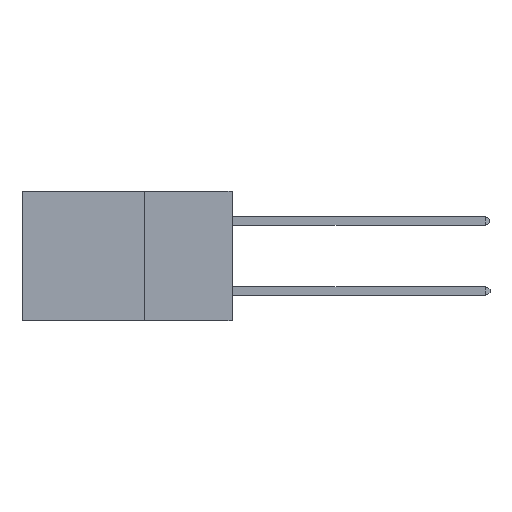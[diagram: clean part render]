
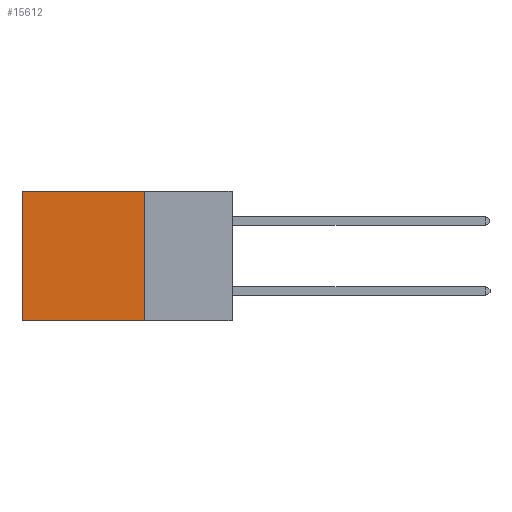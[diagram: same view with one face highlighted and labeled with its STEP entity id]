
A CAD part, left-side view. The second image highlights one B-rep face of the part: STEP entity #15612.
In plain terms, the highlighted planar face has unit normal (-1, 0, 0).
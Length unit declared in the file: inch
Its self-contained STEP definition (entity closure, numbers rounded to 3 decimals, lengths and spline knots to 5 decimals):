
#916 = VECTOR ( 'NONE', #1534, 39.37008 ) ;
#1534 = DIRECTION ( 'NONE',  ( 0., 0., -1. ) ) ;
#1801 = ORIENTED_EDGE ( 'NONE', *, *, #16509, .T. ) ;
#2126 = AXIS2_PLACEMENT_3D ( 'NONE', #10217, #15473, #5063 ) ;
#3080 = CARTESIAN_POINT ( 'NONE',  ( 0.2875, 0.6, 0. ) ) ;
#4008 = VERTEX_POINT ( 'NONE', #3080 ) ;
#4087 = CARTESIAN_POINT ( 'NONE',  ( 0.2875, 0.25, 0. ) ) ;
#4683 = DIRECTION ( 'NONE',  ( 0., 0., -1. ) ) ;
#5063 = DIRECTION ( 'NONE',  ( 0., 0., -1. ) ) ;
#5077 = LINE ( 'NONE', #11322, #12059 ) ;
#5838 = LINE ( 'NONE', #20955, #916 ) ;
#6057 = VERTEX_POINT ( 'NONE', #19304 ) ;
#8002 = FACE_OUTER_BOUND ( 'NONE', #17162, .T. ) ;
#8270 = VERTEX_POINT ( 'NONE', #15749 ) ;
#8512 = PLANE ( 'NONE',  #2126 ) ;
#8953 = ORIENTED_EDGE ( 'NONE', *, *, #21333, .F. ) ;
#9000 = ORIENTED_EDGE ( 'NONE', *, *, #22666, .T. ) ;
#9017 = LINE ( 'NONE', #4087, #13585 ) ;
#10217 = CARTESIAN_POINT ( 'NONE',  ( 0.2875, 0.25, 0. ) ) ;
#11005 = DIRECTION ( 'NONE',  ( 0., 1., 0. ) ) ;
#11295 = ORIENTED_EDGE ( 'NONE', *, *, #18856, .F. ) ;
#11322 = CARTESIAN_POINT ( 'NONE',  ( 0.2875, 0.25, -0.37 ) ) ;
#11631 = VERTEX_POINT ( 'NONE', #21546 ) ;
#11817 = VECTOR ( 'NONE', #4683, 39.37008 ) ;
#12059 = VECTOR ( 'NONE', #13052, 39.37008 ) ;
#13052 = DIRECTION ( 'NONE',  ( 0., 1., 0. ) ) ;
#13585 = VECTOR ( 'NONE', #11005, 39.37008 ) ;
#15024 = CARTESIAN_POINT ( 'NONE',  ( 0.2875, 0.25, 0. ) ) ;
#15473 = DIRECTION ( 'NONE',  ( 1., 0., 0. ) ) ;
#15612 = ADVANCED_FACE ( 'NONE', ( #8002 ), #8512, .F. ) ;
#15749 = CARTESIAN_POINT ( 'NONE',  ( 0.2875, 0.6, -0.37 ) ) ;
#16509 = EDGE_CURVE ( 'NONE', #6057, #4008, #9017, .T. ) ;
#17162 = EDGE_LOOP ( 'NONE', ( #9000, #8953, #11295, #1801 ) ) ;
#18856 = EDGE_CURVE ( 'NONE', #6057, #11631, #21251, .T. ) ;
#19304 = CARTESIAN_POINT ( 'NONE',  ( 0.2875, 0.25, 0. ) ) ;
#20955 = CARTESIAN_POINT ( 'NONE',  ( 0.2875, 0.6, 0. ) ) ;
#21251 = LINE ( 'NONE', #15024, #11817 ) ;
#21333 = EDGE_CURVE ( 'NONE', #11631, #8270, #5077, .T. ) ;
#21546 = CARTESIAN_POINT ( 'NONE',  ( 0.2875, 0.25, -0.37 ) ) ;
#22666 = EDGE_CURVE ( 'NONE', #4008, #8270, #5838, .T. ) ;
